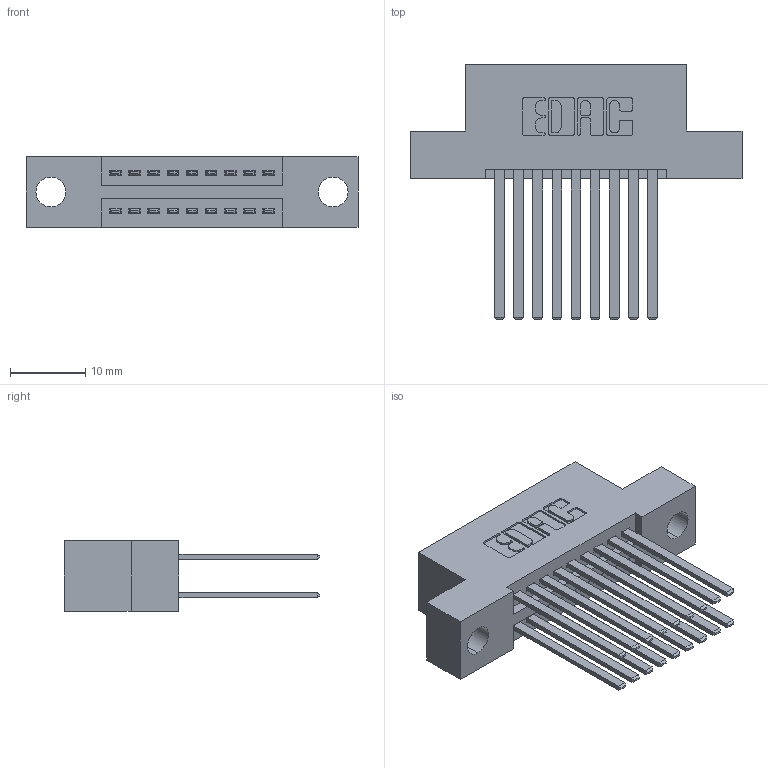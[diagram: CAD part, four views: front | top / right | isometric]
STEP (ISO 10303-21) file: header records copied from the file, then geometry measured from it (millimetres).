
FILE_DESCRIPTION (( 'STEP AP203' ), '1' );
FILE_NAME ('395-018-544-204.STEP', '2021-06-14T18:36:30', ( '' ), ( '' ), 'SwSTEP 2.0', 'SolidWorks 2020', '' );
FILE_SCHEMA (( 'CONFIG_CONTROL_DESIGN' ));
Length unit declared in the file: inch
Products named in the file (3): 395-018-544-204; 345-292-001_345-293-144; 345 Part_Flush Mounting Lugs - 0.156 Dia-TI
Assembly tree (19 placements, depth 2):
  395-018-544-204
    345 Part_Flush Mounting Lugs - 0.156 Dia-TI
    345-292-001_345-293-144  x18
Bounding box: 44.07 x 33.96 x 9.4 mm (x, y, z)
Volume: 4121 mm3; surface area: 6043.5 mm2
Topology: 19 solids, 19 shells, 932 faces, 2735 edges, 1798 vertices
Faces by surface type: plane 616, cylinder 316
Entity records: 11739 total; most frequent: CARTESIAN_POINT 2002, ORIENTED_EDGE 1934, DIRECTION 1803, EDGE_CURVE 967, LINE 803, VECTOR 803, VERTEX_POINT 642, AXIS2_PLACEMENT_3D 500
